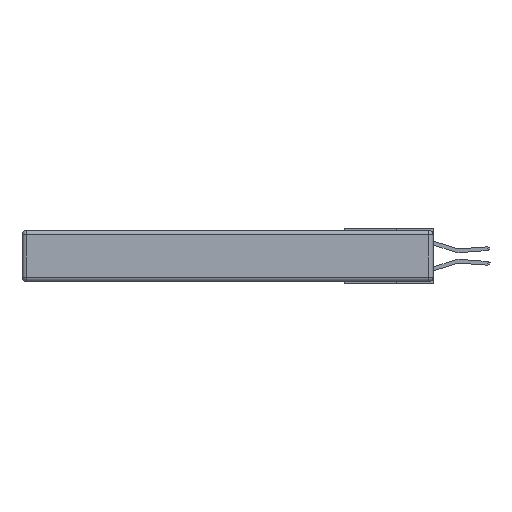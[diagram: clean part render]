
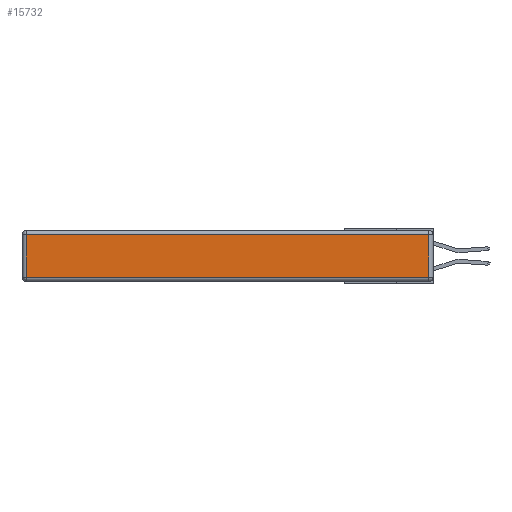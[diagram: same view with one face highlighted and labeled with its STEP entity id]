
A CAD part, left-side view. The second image highlights one B-rep face of the part: STEP entity #15732.
In plain terms, the highlighted planar face has unit normal (-1, 0, 0).
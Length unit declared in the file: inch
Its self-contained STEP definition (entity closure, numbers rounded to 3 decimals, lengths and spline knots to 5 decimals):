
#1891 = VECTOR ( 'NONE', #22869, 39.37008 ) ;
#2211 = CARTESIAN_POINT ( 'NONE',  ( 0., 0., -0.313 ) ) ;
#2285 = AXIS2_PLACEMENT_3D ( 'NONE', #22059, #24519, #12053 ) ;
#2548 = LINE ( 'NONE', #2211, #25849 ) ;
#2912 = EDGE_LOOP ( 'NONE', ( #22441, #22923, #3635, #4050 ) ) ;
#3635 = ORIENTED_EDGE ( 'NONE', *, *, #15490, .T. ) ;
#4050 = ORIENTED_EDGE ( 'NONE', *, *, #27915, .T. ) ;
#4072 = DIRECTION ( 'NONE',  ( 0., 0., 1. ) ) ;
#6158 = FACE_OUTER_BOUND ( 'NONE', #2912, .T. ) ;
#6549 = VERTEX_POINT ( 'NONE', #18369 ) ;
#8378 = EDGE_CURVE ( 'NONE', #6549, #25552, #13503, .T. ) ;
#10754 = CARTESIAN_POINT ( 'NONE',  ( 0., 0.03, -0.03 ) ) ;
#11490 = CARTESIAN_POINT ( 'NONE',  ( 0., 2.72, -0.313 ) ) ;
#12053 = DIRECTION ( 'NONE',  ( 0., 0., 1. ) ) ;
#12115 = CARTESIAN_POINT ( 'NONE',  ( 0., 2.72, -0.03 ) ) ;
#12663 = VECTOR ( 'NONE', #18838, 39.37008 ) ;
#12894 = EDGE_CURVE ( 'NONE', #23592, #6549, #2548, .T. ) ;
#13503 = LINE ( 'NONE', #30941, #24935 ) ;
#14701 = PLANE ( 'NONE',  #2285 ) ;
#15490 = EDGE_CURVE ( 'NONE', #25552, #19369, #16831, .T. ) ;
#15732 = ADVANCED_FACE ( 'NONE', ( #6158 ), #14701, .T. ) ;
#16831 = LINE ( 'NONE', #18729, #12663 ) ;
#18369 = CARTESIAN_POINT ( 'NONE',  ( 0., 0.03, -0.313 ) ) ;
#18729 = CARTESIAN_POINT ( 'NONE',  ( 0., 2.75, -0.03 ) ) ;
#18838 = DIRECTION ( 'NONE',  ( 0., 1., 0. ) ) ;
#19369 = VERTEX_POINT ( 'NONE', #12115 ) ;
#19825 = LINE ( 'NONE', #20198, #1891 ) ;
#20198 = CARTESIAN_POINT ( 'NONE',  ( 0., 2.72, -0.343 ) ) ;
#21941 = DIRECTION ( 'NONE',  ( 0., -1., 0. ) ) ;
#22059 = CARTESIAN_POINT ( 'NONE',  ( 0., 0., -0.343 ) ) ;
#22441 = ORIENTED_EDGE ( 'NONE', *, *, #12894, .T. ) ;
#22869 = DIRECTION ( 'NONE',  ( 0., 0., -1. ) ) ;
#22923 = ORIENTED_EDGE ( 'NONE', *, *, #8378, .T. ) ;
#23592 = VERTEX_POINT ( 'NONE', #11490 ) ;
#24519 = DIRECTION ( 'NONE',  ( -1., 0., 0. ) ) ;
#24935 = VECTOR ( 'NONE', #4072, 39.37008 ) ;
#25552 = VERTEX_POINT ( 'NONE', #10754 ) ;
#25849 = VECTOR ( 'NONE', #21941, 39.37008 ) ;
#27915 = EDGE_CURVE ( 'NONE', #19369, #23592, #19825, .T. ) ;
#30941 = CARTESIAN_POINT ( 'NONE',  ( 0., 0.03, -0.343 ) ) ;
